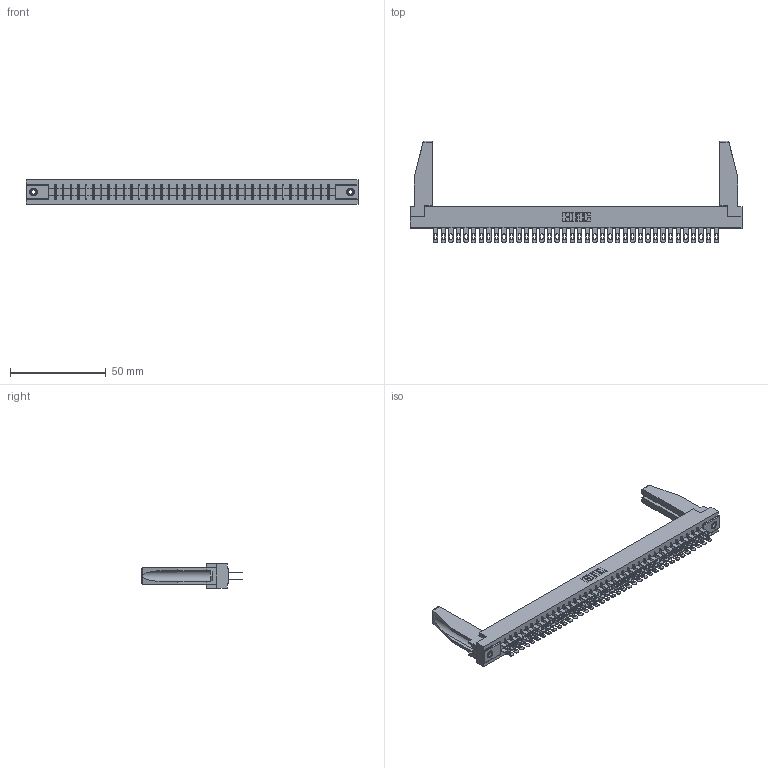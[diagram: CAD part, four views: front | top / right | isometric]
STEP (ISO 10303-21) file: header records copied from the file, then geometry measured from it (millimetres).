
FILE_DESCRIPTION (( 'STEP AP203' ), '1' );
FILE_NAME ('315-076-500-278.STEP', '2019-09-10T22:22:43', ( '' ), ( '' ), 'SwSTEP 2.0', 'SolidWorks 2016', '' );
FILE_SCHEMA (( 'CONFIG_CONTROL_DESIGN' ));
Length unit declared in the file: inch
Products named in the file (5): 305-290-001_500; 315-076-500-278; 345-250-001_345-250-001-102; 307-220-078; 305 Part_.156 Dia
Assembly tree (81 placements, depth 2):
  315-076-500-278
    305 Part_.156 Dia
    305-290-001_500  x76
    345-250-001_345-250-001-102  x2
    307-220-078  x2
Bounding box: 173.58 x 52.88 x 12.7 mm (x, y, z)
Volume: 22315 mm3; surface area: 28527.5 mm2
Topology: 81 solids, 81 shells, 4046 faces, 11552 edges, 7488 vertices
Faces by surface type: plane 2280, cylinder 1598, sphere 152, cone 12, torus 4
Entity records: 44092 total; most frequent: CARTESIAN_POINT 7302, ORIENTED_EDGE 7206, DIRECTION 7027, EDGE_CURVE 3603, LINE 2905, VECTOR 2905, VERTEX_POINT 2294, AXIS2_PLACEMENT_3D 2061
